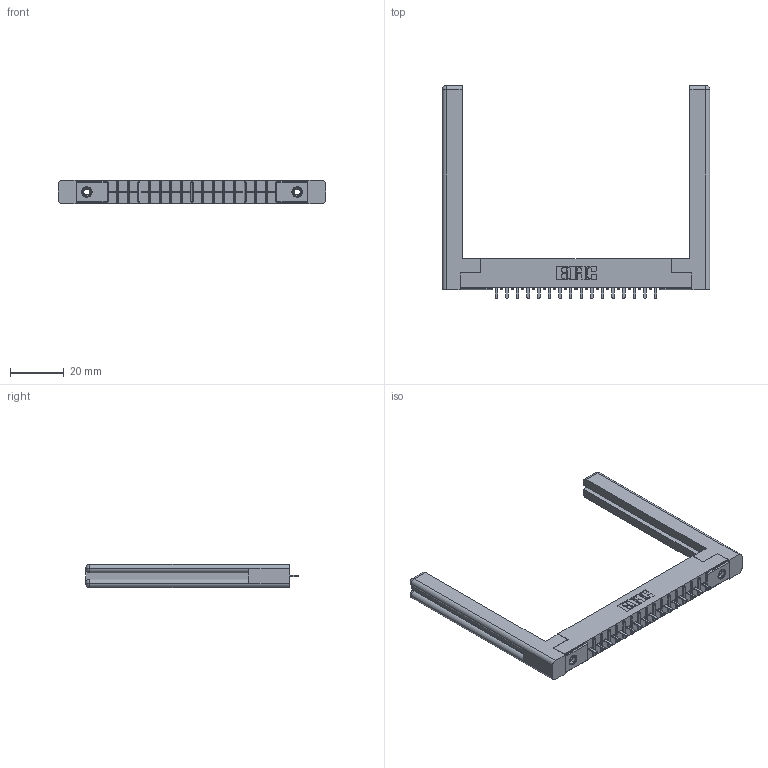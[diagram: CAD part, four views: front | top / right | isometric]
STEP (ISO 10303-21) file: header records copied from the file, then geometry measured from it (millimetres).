
FILE_DESCRIPTION (( 'STEP AP203' ), '1' );
FILE_NAME ('356-016-421-158.STEP', '2020-09-23T12:46:24', ( '' ), ( '' ), 'SwSTEP 2.0', 'SolidWorks 2020', '' );
FILE_SCHEMA (( 'CONFIG_CONTROL_DESIGN' ));
Length unit declared in the file: inch
Products named in the file (5): 356-016-421-158; 307-220-058; 306-290-001_121; 345-250-001_345-250-001-102; 306 Part_.156 Dia
Assembly tree (21 placements, depth 2):
  356-016-421-158
    306 Part_.156 Dia
    306-290-001_121  x16
    345-250-001_345-250-001-102  x2
    307-220-058  x2
Bounding box: 100.03 x 79.53 x 8.71 mm (x, y, z)
Volume: 14435.9 mm3; surface area: 15038.7 mm2
Topology: 21 solids, 21 shells, 1378 faces, 3822 edges, 2448 vertices
Faces by surface type: plane 904, cylinder 386, sphere 64, cone 12, torus 12
Entity records: 20878 total; most frequent: CARTESIAN_POINT 3510, DIRECTION 3419, ORIENTED_EDGE 3418, EDGE_CURVE 1709, LINE 1317, VECTOR 1317, VERTEX_POINT 1088, AXIS2_PLACEMENT_3D 1051
